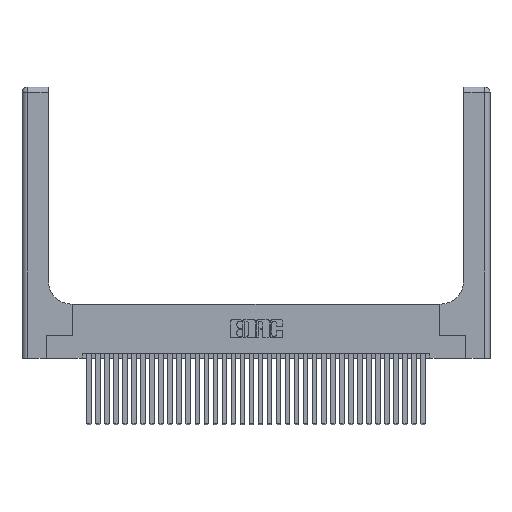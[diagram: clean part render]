
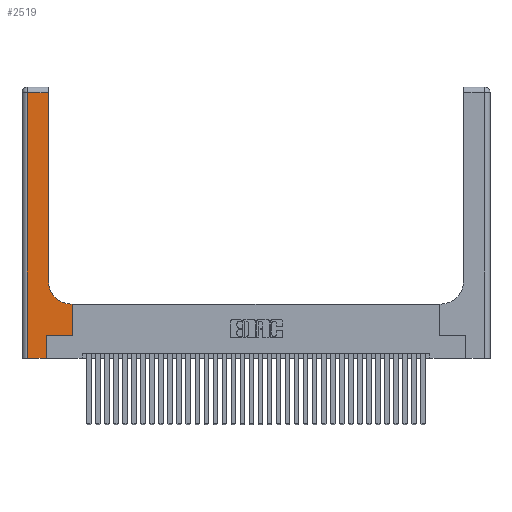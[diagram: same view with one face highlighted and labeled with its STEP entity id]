
A CAD part, top view. The second image highlights one B-rep face of the part: STEP entity #2519.
In plain terms, the highlighted planar face has unit normal (0, 0, 1).
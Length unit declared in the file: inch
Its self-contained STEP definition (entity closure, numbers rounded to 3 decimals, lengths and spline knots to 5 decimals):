
#40 = VECTOR ( 'NONE', #11760, 39.37008 ) ;
#242 = VECTOR ( 'NONE', #1441, 39.37008 ) ;
#496 = EDGE_CURVE ( 'NONE', #20886, #10844, #30809, .T. ) ;
#932 = EDGE_CURVE ( 'NONE', #5936, #20886, #32947, .T. ) ;
#1441 = DIRECTION ( 'NONE',  ( 0., 1., 0. ) ) ;
#2519 = ADVANCED_FACE ( 'NONE', ( #25164 ), #4157, .F. ) ;
#3191 = LINE ( 'NONE', #28837, #25335 ) ;
#3426 = CARTESIAN_POINT ( 'NONE',  ( 0., 0., 0.37 ) ) ;
#3682 = VERTEX_POINT ( 'NONE', #22068 ) ;
#4157 = PLANE ( 'NONE',  #10550 ) ;
#4341 = CARTESIAN_POINT ( 'NONE',  ( 0.2915, 2.94, 0.37 ) ) ;
#5371 = CARTESIAN_POINT ( 'NONE',  ( 0.269, 0., 0.37 ) ) ;
#5936 = VERTEX_POINT ( 'NONE', #24399 ) ;
#6371 = VERTEX_POINT ( 'NONE', #28494 ) ;
#6647 = DIRECTION ( 'NONE',  ( 0., 1., 0. ) ) ;
#7927 = CARTESIAN_POINT ( 'NONE',  ( 0.5415, 0.85, 0.37 ) ) ;
#8044 = DIRECTION ( 'NONE',  ( 1., 0., 0. ) ) ;
#8100 = DIRECTION ( 'NONE',  ( -1., 0., 0. ) ) ;
#9286 = VERTEX_POINT ( 'NONE', #35094 ) ;
#10437 = EDGE_CURVE ( 'NONE', #3682, #5936, #34583, .T. ) ;
#10550 = AXIS2_PLACEMENT_3D ( 'NONE', #15266, #29074, #12623 ) ;
#10671 = DIRECTION ( 'NONE',  ( 0., 0., -1. ) ) ;
#10844 = VERTEX_POINT ( 'NONE', #15614 ) ;
#11433 = ORIENTED_EDGE ( 'NONE', *, *, #20491, .T. ) ;
#11600 = CARTESIAN_POINT ( 'NONE',  ( 0.2915, 0.85, 0.37 ) ) ;
#11760 = DIRECTION ( 'NONE',  ( 1., 0., 0. ) ) ;
#12623 = DIRECTION ( 'NONE',  ( -1., 0., 0. ) ) ;
#12686 = DIRECTION ( 'NONE',  ( 0., 1., 0. ) ) ;
#14452 = CIRCLE ( 'NONE', #17952, 0.25 ) ;
#14991 = VERTEX_POINT ( 'NONE', #32373 ) ;
#15145 = DIRECTION ( 'NONE',  ( 1., 0., 0. ) ) ;
#15266 = CARTESIAN_POINT ( 'NONE',  ( 0., 3., 0.37 ) ) ;
#15498 = VERTEX_POINT ( 'NONE', #11600 ) ;
#15614 = CARTESIAN_POINT ( 'NONE',  ( 0.269, 0.25, 0.37 ) ) ;
#16080 = DIRECTION ( 'NONE',  ( -1., 0., 0. ) ) ;
#16255 = EDGE_CURVE ( 'NONE', #15498, #27855, #20775, .T. ) ;
#16632 = VECTOR ( 'NONE', #18263, 39.37008 ) ;
#16880 = LINE ( 'NONE', #31125, #29301 ) ;
#17645 = CARTESIAN_POINT ( 'NONE',  ( 0.2915, 3., 0.37 ) ) ;
#17925 = ORIENTED_EDGE ( 'NONE', *, *, #16255, .T. ) ;
#17952 = AXIS2_PLACEMENT_3D ( 'NONE', #7927, #10671, #8044 ) ;
#18145 = CARTESIAN_POINT ( 'NONE',  ( 0.06, 3., 0.37 ) ) ;
#18263 = DIRECTION ( 'NONE',  ( 0., -1., 0. ) ) ;
#20491 = EDGE_CURVE ( 'NONE', #6371, #15498, #14452, .T. ) ;
#20775 = LINE ( 'NONE', #17645, #242 ) ;
#20886 = VERTEX_POINT ( 'NONE', #22977 ) ;
#21364 = EDGE_CURVE ( 'NONE', #10844, #14991, #16880, .T. ) ;
#21564 = ORIENTED_EDGE ( 'NONE', *, *, #22336, .T. ) ;
#21649 = CARTESIAN_POINT ( 'NONE',  ( 0.2915, 0.6, 0.37 ) ) ;
#22068 = CARTESIAN_POINT ( 'NONE',  ( 0.06, 2.94, 0.37 ) ) ;
#22336 = EDGE_CURVE ( 'NONE', #14991, #9286, #3191, .T. ) ;
#22383 = ORIENTED_EDGE ( 'NONE', *, *, #932, .T. ) ;
#22977 = CARTESIAN_POINT ( 'NONE',  ( 0.269, 0., 0.37 ) ) ;
#24399 = CARTESIAN_POINT ( 'NONE',  ( 0.06, 0., 0.37 ) ) ;
#25164 = FACE_OUTER_BOUND ( 'NONE', #27381, .T. ) ;
#25335 = VECTOR ( 'NONE', #6647, 39.37008 ) ;
#26002 = ORIENTED_EDGE ( 'NONE', *, *, #34524, .T. ) ;
#26008 = VECTOR ( 'NONE', #8100, 39.37008 ) ;
#26097 = VECTOR ( 'NONE', #12686, 39.37008 ) ;
#27199 = ORIENTED_EDGE ( 'NONE', *, *, #10437, .T. ) ;
#27381 = EDGE_LOOP ( 'NONE', ( #17925, #26002, #27199, #22383, #34645, #32262, #21564, #27410, #11433 ) ) ;
#27410 = ORIENTED_EDGE ( 'NONE', *, *, #27431, .T. ) ;
#27431 = EDGE_CURVE ( 'NONE', #9286, #6371, #34836, .T. ) ;
#27855 = VERTEX_POINT ( 'NONE', #4341 ) ;
#28494 = CARTESIAN_POINT ( 'NONE',  ( 0.5415, 0.6, 0.37 ) ) ;
#28837 = CARTESIAN_POINT ( 'NONE',  ( 0.5585, 0.25, 0.37 ) ) ;
#29074 = DIRECTION ( 'NONE',  ( 0., 0., -1. ) ) ;
#29301 = VECTOR ( 'NONE', #15145, 39.37008 ) ;
#29870 = LINE ( 'NONE', #32584, #26008 ) ;
#30809 = LINE ( 'NONE', #5371, #26097 ) ;
#30979 = VECTOR ( 'NONE', #16080, 39.37008 ) ;
#31125 = CARTESIAN_POINT ( 'NONE',  ( 0.269, 0.25, 0.37 ) ) ;
#32262 = ORIENTED_EDGE ( 'NONE', *, *, #21364, .T. ) ;
#32373 = CARTESIAN_POINT ( 'NONE',  ( 0.5585, 0.25, 0.37 ) ) ;
#32584 = CARTESIAN_POINT ( 'NONE',  ( 0., 2.94, 0.37 ) ) ;
#32947 = LINE ( 'NONE', #3426, #40 ) ;
#34524 = EDGE_CURVE ( 'NONE', #27855, #3682, #29870, .T. ) ;
#34583 = LINE ( 'NONE', #18145, #16632 ) ;
#34645 = ORIENTED_EDGE ( 'NONE', *, *, #496, .T. ) ;
#34836 = LINE ( 'NONE', #21649, #30979 ) ;
#35094 = CARTESIAN_POINT ( 'NONE',  ( 0.5585, 0.6, 0.37 ) ) ;
